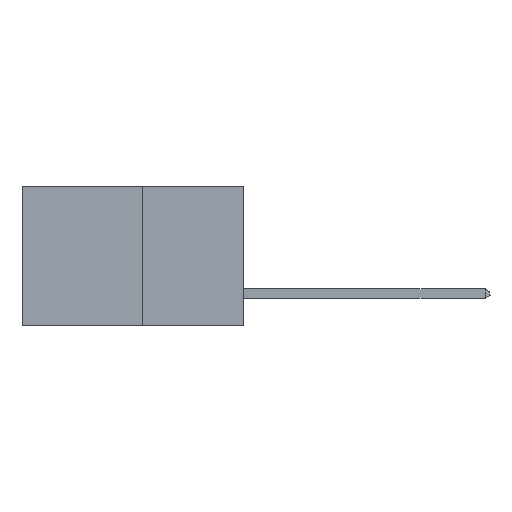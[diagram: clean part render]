
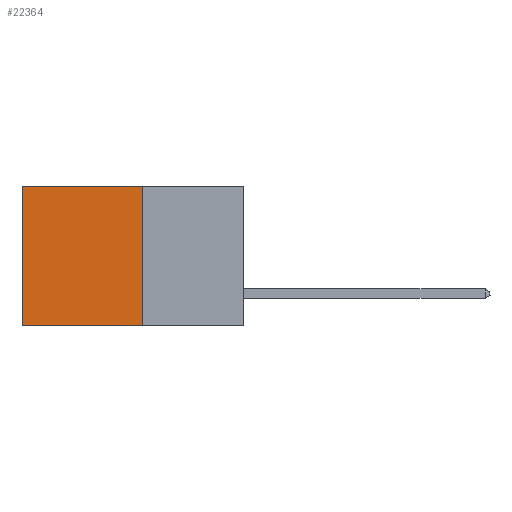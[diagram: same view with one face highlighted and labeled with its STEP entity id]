
A CAD part, left-side view. The second image highlights one B-rep face of the part: STEP entity #22364.
In plain terms, the highlighted planar face has unit normal (-1, 0, 0).
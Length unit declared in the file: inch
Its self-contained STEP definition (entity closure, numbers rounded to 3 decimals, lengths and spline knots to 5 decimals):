
#183 = VERTEX_POINT ( 'NONE', #27190 ) ;
#986 = ORIENTED_EDGE ( 'NONE', *, *, #22353, .T. ) ;
#1533 = DIRECTION ( 'NONE',  ( 0., 1., 0. ) ) ;
#4181 = ORIENTED_EDGE ( 'NONE', *, *, #31056, .T. ) ;
#8152 = CARTESIAN_POINT ( 'NONE',  ( 0.277, 0.59, 0. ) ) ;
#9101 = EDGE_LOOP ( 'NONE', ( #4181, #16445, #15645, #986 ) ) ;
#9144 = CARTESIAN_POINT ( 'NONE',  ( 0.277, 0.27, -0.37 ) ) ;
#10479 = DIRECTION ( 'NONE',  ( 1., 0., 0. ) ) ;
#11361 = CARTESIAN_POINT ( 'NONE',  ( 0.277, 0.27, -0.37 ) ) ;
#11812 = FACE_OUTER_BOUND ( 'NONE', #9101, .T. ) ;
#15645 = ORIENTED_EDGE ( 'NONE', *, *, #15715, .F. ) ;
#15715 = EDGE_CURVE ( 'NONE', #22079, #20327, #25479, .T. ) ;
#16445 = ORIENTED_EDGE ( 'NONE', *, *, #17802, .F. ) ;
#17584 = CARTESIAN_POINT ( 'NONE',  ( 0.277, 0.27, 0. ) ) ;
#17692 = DIRECTION ( 'NONE',  ( 0., 1., 0. ) ) ;
#17802 = EDGE_CURVE ( 'NONE', #20327, #183, #22127, .T. ) ;
#17846 = DIRECTION ( 'NONE',  ( 0., 0., -1. ) ) ;
#18701 = AXIS2_PLACEMENT_3D ( 'NONE', #27606, #10479, #27717 ) ;
#19163 = VERTEX_POINT ( 'NONE', #8152 ) ;
#20327 = VERTEX_POINT ( 'NONE', #29782 ) ;
#21343 = VECTOR ( 'NONE', #1533, 39.37008 ) ;
#22079 = VERTEX_POINT ( 'NONE', #23752 ) ;
#22127 = LINE ( 'NONE', #11361, #21343 ) ;
#22353 = EDGE_CURVE ( 'NONE', #22079, #19163, #25702, .T. ) ;
#22364 = ADVANCED_FACE ( 'NONE', ( #11812 ), #25212, .F. ) ;
#22763 = CARTESIAN_POINT ( 'NONE',  ( 0.277, 0.59, -0.37 ) ) ;
#23752 = CARTESIAN_POINT ( 'NONE',  ( 0.277, 0.27, 0. ) ) ;
#23933 = VECTOR ( 'NONE', #28836, 39.37008 ) ;
#24358 = VECTOR ( 'NONE', #17846, 39.37008 ) ;
#25212 = PLANE ( 'NONE',  #18701 ) ;
#25479 = LINE ( 'NONE', #9144, #23933 ) ;
#25702 = LINE ( 'NONE', #17584, #26488 ) ;
#26488 = VECTOR ( 'NONE', #17692, 39.37008 ) ;
#27190 = CARTESIAN_POINT ( 'NONE',  ( 0.277, 0.59, -0.37 ) ) ;
#27606 = CARTESIAN_POINT ( 'NONE',  ( 0.277, 0.27, -0.37 ) ) ;
#27717 = DIRECTION ( 'NONE',  ( 0., 0., -1. ) ) ;
#28836 = DIRECTION ( 'NONE',  ( 0., 0., -1. ) ) ;
#29782 = CARTESIAN_POINT ( 'NONE',  ( 0.277, 0.27, -0.37 ) ) ;
#31056 = EDGE_CURVE ( 'NONE', #19163, #183, #31677, .T. ) ;
#31677 = LINE ( 'NONE', #22763, #24358 ) ;
